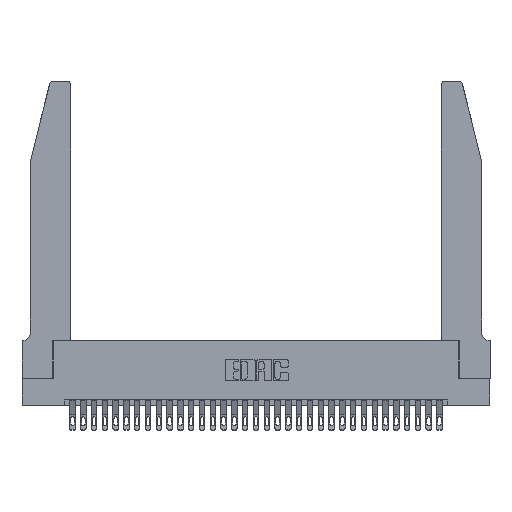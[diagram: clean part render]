
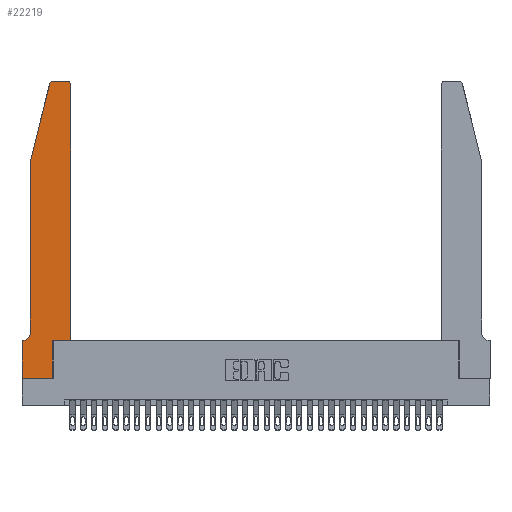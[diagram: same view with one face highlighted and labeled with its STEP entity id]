
A CAD part, top view. The second image highlights one B-rep face of the part: STEP entity #22219.
In plain terms, the highlighted planar face has unit normal (0, 0, 1).
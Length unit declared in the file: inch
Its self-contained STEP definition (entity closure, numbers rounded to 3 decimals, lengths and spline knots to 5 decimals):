
#1319 = AXIS2_PLACEMENT_3D ( 'NONE', #13287, #31118, #15866 ) ;
#1720 = CARTESIAN_POINT ( 'NONE',  ( 0., 0., 0.37 ) ) ;
#1804 = CARTESIAN_POINT ( 'NONE',  ( 0.4505, 0.35, 0.37 ) ) ;
#2019 = LINE ( 'NONE', #20708, #21998 ) ;
#2369 = CARTESIAN_POINT ( 'NONE',  ( 0.4505, 2.72, 0.37 ) ) ;
#2857 = EDGE_CURVE ( 'NONE', #22464, #25930, #25088, .T. ) ;
#2988 = DIRECTION ( 'NONE',  ( 0., 1., 0. ) ) ;
#3174 = VERTEX_POINT ( 'NONE', #2369 ) ;
#3182 = EDGE_CURVE ( 'NONE', #26464, #10179, #22302, .T. ) ;
#3623 = VECTOR ( 'NONE', #14216, 39.37008 ) ;
#4671 = VECTOR ( 'NONE', #2988, 39.37008 ) ;
#5041 = CARTESIAN_POINT ( 'NONE',  ( 0., 0., 0.37 ) ) ;
#5468 = ORIENTED_EDGE ( 'NONE', *, *, #31733, .T. ) ;
#5552 = CARTESIAN_POINT ( 'NONE',  ( 0.0755, 0.35, 0.37 ) ) ;
#5649 = VERTEX_POINT ( 'NONE', #30854 ) ;
#5681 = CARTESIAN_POINT ( 'NONE',  ( 0.4205, 2.75, 0.37 ) ) ;
#6111 = ORIENTED_EDGE ( 'NONE', *, *, #3182, .T. ) ;
#6467 = CARTESIAN_POINT ( 'NONE',  ( 0.25487, 2.72718, 0.37 ) ) ;
#6504 = LINE ( 'NONE', #13449, #19478 ) ;
#6946 = CARTESIAN_POINT ( 'NONE',  ( 0., 0.35, 0.37 ) ) ;
#7057 = DIRECTION ( 'NONE',  ( 0., 0., 1. ) ) ;
#8205 = CIRCLE ( 'NONE', #12381, 0.07 ) ;
#8292 = VERTEX_POINT ( 'NONE', #12941 ) ;
#9020 = VECTOR ( 'NONE', #11457, 39.37008 ) ;
#9244 = CARTESIAN_POINT ( 'NONE',  ( 0., 0., 0.37 ) ) ;
#9253 = LINE ( 'NONE', #24422, #15348 ) ;
#9376 = CARTESIAN_POINT ( 'NONE',  ( 0.4505, 0.35, 0.37 ) ) ;
#9628 = CARTESIAN_POINT ( 'NONE',  ( 0.2865, 0.35, 0.37 ) ) ;
#10179 = VERTEX_POINT ( 'NONE', #9244 ) ;
#10187 = VECTOR ( 'NONE', #20612, 39.37008 ) ;
#10487 = EDGE_LOOP ( 'NONE', ( #31735, #33195, #29100, #15730, #19972, #5468, #6111, #22658, #30377, #33162, #13337, #22186 ) ) ;
#10708 = CARTESIAN_POINT ( 'NONE',  ( 0.284, 2.75, 0.37 ) ) ;
#10864 = VERTEX_POINT ( 'NONE', #1804 ) ;
#10882 = CARTESIAN_POINT ( 'NONE',  ( 0.4205, 2.72, 0.37 ) ) ;
#11457 = DIRECTION ( 'NONE',  ( 0., 1., 0. ) ) ;
#12381 = AXIS2_PLACEMENT_3D ( 'NONE', #29115, #13810, #31649 ) ;
#12532 = EDGE_CURVE ( 'NONE', #25930, #18664, #27582, .T. ) ;
#12941 = CARTESIAN_POINT ( 'NONE',  ( 0.0755, 2., 0.37 ) ) ;
#13173 = EDGE_CURVE ( 'NONE', #20888, #5649, #8205, .T. ) ;
#13287 = CARTESIAN_POINT ( 'NONE',  ( 0.284, 2.72, 0.37 ) ) ;
#13337 = ORIENTED_EDGE ( 'NONE', *, *, #32729, .T. ) ;
#13449 = CARTESIAN_POINT ( 'NONE',  ( 0.0755, 2., 0.37 ) ) ;
#13504 = DIRECTION ( 'NONE',  ( 1., 0., 0. ) ) ;
#13810 = DIRECTION ( 'NONE',  ( 0., 0., -1. ) ) ;
#14187 = VERTEX_POINT ( 'NONE', #25622 ) ;
#14216 = DIRECTION ( 'NONE',  ( -1., 0., 0. ) ) ;
#15348 = VECTOR ( 'NONE', #32065, 39.37008 ) ;
#15730 = ORIENTED_EDGE ( 'NONE', *, *, #25200, .T. ) ;
#15866 = DIRECTION ( 'NONE',  ( 1., 0., 0. ) ) ;
#15926 = CIRCLE ( 'NONE', #28445, 0.03 ) ;
#16203 = VECTOR ( 'NONE', #22550, 39.37008 ) ;
#16779 = CARTESIAN_POINT ( 'NONE',  ( 0.2605, 2.75, 0.37 ) ) ;
#17387 = PLANE ( 'NONE',  #20210 ) ;
#17886 = EDGE_CURVE ( 'NONE', #3174, #22464, #15926, .T. ) ;
#18005 = EDGE_CURVE ( 'NONE', #14187, #24982, #33056, .T. ) ;
#18664 = VERTEX_POINT ( 'NONE', #6467 ) ;
#19230 = CARTESIAN_POINT ( 'NONE',  ( 0.2865, 0.35, 0.37 ) ) ;
#19478 = VECTOR ( 'NONE', #28757, 39.37008 ) ;
#19972 = ORIENTED_EDGE ( 'NONE', *, *, #13173, .T. ) ;
#20210 = AXIS2_PLACEMENT_3D ( 'NONE', #6946, #7057, #25104 ) ;
#20483 = EDGE_CURVE ( 'NONE', #24982, #10864, #9253, .T. ) ;
#20612 = DIRECTION ( 'NONE',  ( 0., -1., 0. ) ) ;
#20708 = CARTESIAN_POINT ( 'NONE',  ( 0.0755, 2., 0.37 ) ) ;
#20888 = VERTEX_POINT ( 'NONE', #28506 ) ;
#21022 = LINE ( 'NONE', #5552, #27772 ) ;
#21094 = DIRECTION ( 'NONE',  ( -1., 0., 0. ) ) ;
#21998 = VECTOR ( 'NONE', #28371, 39.37008 ) ;
#22186 = ORIENTED_EDGE ( 'NONE', *, *, #17886, .T. ) ;
#22219 = ADVANCED_FACE ( 'NONE', ( #26850 ), #17387, .T. ) ;
#22302 = LINE ( 'NONE', #5041, #10187 ) ;
#22464 = VERTEX_POINT ( 'NONE', #5681 ) ;
#22550 = DIRECTION ( 'NONE',  ( 1., 0., 0. ) ) ;
#22658 = ORIENTED_EDGE ( 'NONE', *, *, #31422, .T. ) ;
#24422 = CARTESIAN_POINT ( 'NONE',  ( 0.4505, 0.35, 0.37 ) ) ;
#24982 = VERTEX_POINT ( 'NONE', #9628 ) ;
#25088 = LINE ( 'NONE', #16779, #3623 ) ;
#25104 = DIRECTION ( 'NONE',  ( 1., 0., 0. ) ) ;
#25200 = EDGE_CURVE ( 'NONE', #8292, #20888, #2019, .T. ) ;
#25315 = LINE ( 'NONE', #9376, #4671 ) ;
#25622 = CARTESIAN_POINT ( 'NONE',  ( 0.2865, 0., 0.37 ) ) ;
#25930 = VERTEX_POINT ( 'NONE', #10708 ) ;
#26464 = VERTEX_POINT ( 'NONE', #30706 ) ;
#26850 = FACE_OUTER_BOUND ( 'NONE', #10487, .T. ) ;
#27370 = EDGE_CURVE ( 'NONE', #18664, #8292, #6504, .T. ) ;
#27582 = CIRCLE ( 'NONE', #1319, 0.03 ) ;
#27772 = VECTOR ( 'NONE', #21094, 39.37008 ) ;
#28371 = DIRECTION ( 'NONE',  ( 0., -1., 0. ) ) ;
#28445 = AXIS2_PLACEMENT_3D ( 'NONE', #10882, #28826, #13504 ) ;
#28506 = CARTESIAN_POINT ( 'NONE',  ( 0.0755, 0.42, 0.37 ) ) ;
#28757 = DIRECTION ( 'NONE',  ( -0.239, -0.971, 0. ) ) ;
#28826 = DIRECTION ( 'NONE',  ( 0., 0., 1. ) ) ;
#29100 = ORIENTED_EDGE ( 'NONE', *, *, #27370, .T. ) ;
#29115 = CARTESIAN_POINT ( 'NONE',  ( 0.0055, 0.42, 0.37 ) ) ;
#29757 = LINE ( 'NONE', #1720, #16203 ) ;
#30377 = ORIENTED_EDGE ( 'NONE', *, *, #18005, .T. ) ;
#30706 = CARTESIAN_POINT ( 'NONE',  ( 0., 0.35, 0.37 ) ) ;
#30854 = CARTESIAN_POINT ( 'NONE',  ( 0.0055, 0.35, 0.37 ) ) ;
#31118 = DIRECTION ( 'NONE',  ( 0., 0., 1. ) ) ;
#31422 = EDGE_CURVE ( 'NONE', #10179, #14187, #29757, .T. ) ;
#31649 = DIRECTION ( 'NONE',  ( -1., 0., 0. ) ) ;
#31733 = EDGE_CURVE ( 'NONE', #5649, #26464, #21022, .T. ) ;
#31735 = ORIENTED_EDGE ( 'NONE', *, *, #2857, .T. ) ;
#32065 = DIRECTION ( 'NONE',  ( 1., 0., 0. ) ) ;
#32729 = EDGE_CURVE ( 'NONE', #10864, #3174, #25315, .T. ) ;
#33056 = LINE ( 'NONE', #19230, #9020 ) ;
#33162 = ORIENTED_EDGE ( 'NONE', *, *, #20483, .T. ) ;
#33195 = ORIENTED_EDGE ( 'NONE', *, *, #12532, .T. ) ;
